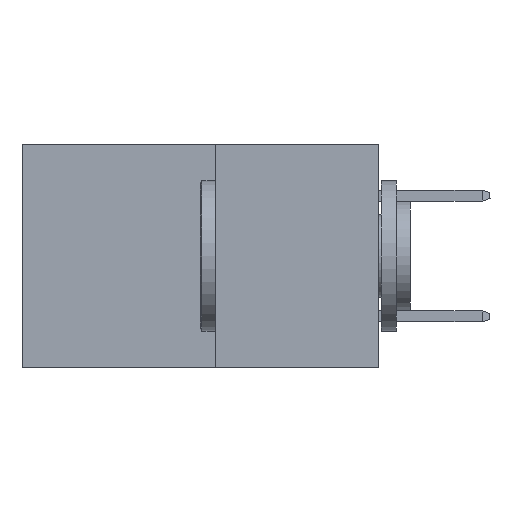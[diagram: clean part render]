
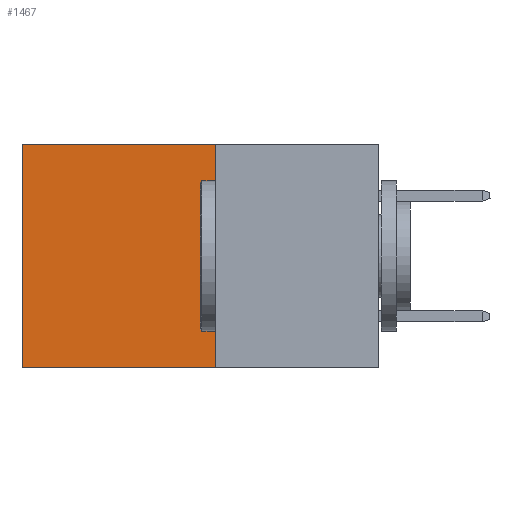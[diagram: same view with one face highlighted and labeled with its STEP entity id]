
A CAD part, left-side view. The second image highlights one B-rep face of the part: STEP entity #1467.
In plain terms, the highlighted planar face has unit normal (-1, 0, 0).
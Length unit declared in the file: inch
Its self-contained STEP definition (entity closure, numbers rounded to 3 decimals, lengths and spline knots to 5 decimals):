
#379 = ORIENTED_EDGE ( 'NONE', *, *, #1024, .T. ) ;
#458 = LINE ( 'NONE', #8639, #2362 ) ;
#885 = VERTEX_POINT ( 'NONE', #8406 ) ;
#1024 = EDGE_CURVE ( 'NONE', #5773, #885, #4245, .T. ) ;
#1113 = FACE_OUTER_BOUND ( 'NONE', #1896, .T. ) ;
#1146 = DIRECTION ( 'NONE',  ( 0., 0., -1. ) ) ;
#1222 = CARTESIAN_POINT ( 'NONE',  ( 0.277, 0.27, -0.37 ) ) ;
#1467 = ADVANCED_FACE ( 'NONE', ( #1113 ), #6920, .F. ) ;
#1802 = DIRECTION ( 'NONE',  ( 1., 0., 0. ) ) ;
#1835 = DIRECTION ( 'NONE',  ( 0., 0., -1. ) ) ;
#1896 = EDGE_LOOP ( 'NONE', ( #7396, #6458, #4434, #379 ) ) ;
#2203 = DIRECTION ( 'NONE',  ( 0., 1., 0. ) ) ;
#2353 = EDGE_CURVE ( 'NONE', #5773, #9023, #8970, .T. ) ;
#2362 = VECTOR ( 'NONE', #2203, 39.37008 ) ;
#2675 = VECTOR ( 'NONE', #4551, 39.37008 ) ;
#3246 = CARTESIAN_POINT ( 'NONE',  ( 0.277, 0.27, -0.37 ) ) ;
#3318 = VECTOR ( 'NONE', #1146, 39.37008 ) ;
#4245 = LINE ( 'NONE', #7529, #2675 ) ;
#4434 = ORIENTED_EDGE ( 'NONE', *, *, #2353, .F. ) ;
#4551 = DIRECTION ( 'NONE',  ( 0., 1., 0. ) ) ;
#5065 = CARTESIAN_POINT ( 'NONE',  ( 0.277, 0.59, -0.37 ) ) ;
#5591 = CARTESIAN_POINT ( 'NONE',  ( 0.277, 0.27, 0. ) ) ;
#5773 = VERTEX_POINT ( 'NONE', #5591 ) ;
#5830 = DIRECTION ( 'NONE',  ( 0., 0., -1. ) ) ;
#6248 = CARTESIAN_POINT ( 'NONE',  ( 0.277, 0.27, -0.37 ) ) ;
#6398 = AXIS2_PLACEMENT_3D ( 'NONE', #3246, #1802, #1835 ) ;
#6458 = ORIENTED_EDGE ( 'NONE', *, *, #9442, .F. ) ;
#6920 = PLANE ( 'NONE',  #6398 ) ;
#7375 = LINE ( 'NONE', #5065, #9376 ) ;
#7396 = ORIENTED_EDGE ( 'NONE', *, *, #8466, .T. ) ;
#7529 = CARTESIAN_POINT ( 'NONE',  ( 0.277, 0.27, 0. ) ) ;
#8406 = CARTESIAN_POINT ( 'NONE',  ( 0.277, 0.59, 0. ) ) ;
#8466 = EDGE_CURVE ( 'NONE', #885, #8868, #7375, .T. ) ;
#8639 = CARTESIAN_POINT ( 'NONE',  ( 0.277, 0.27, -0.37 ) ) ;
#8849 = CARTESIAN_POINT ( 'NONE',  ( 0.277, 0.59, -0.37 ) ) ;
#8868 = VERTEX_POINT ( 'NONE', #8849 ) ;
#8970 = LINE ( 'NONE', #1222, #3318 ) ;
#9023 = VERTEX_POINT ( 'NONE', #6248 ) ;
#9376 = VECTOR ( 'NONE', #5830, 39.37008 ) ;
#9442 = EDGE_CURVE ( 'NONE', #9023, #8868, #458, .T. ) ;
